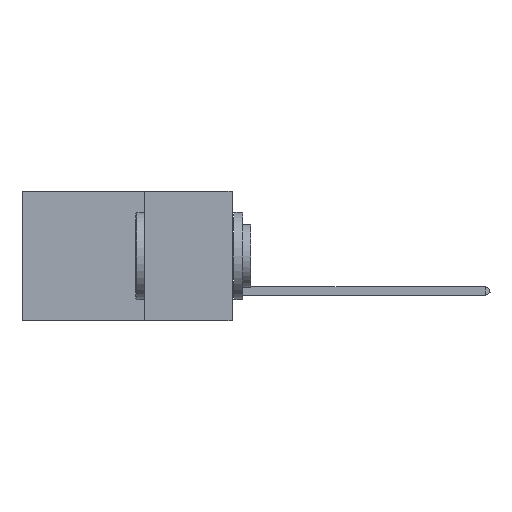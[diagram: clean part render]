
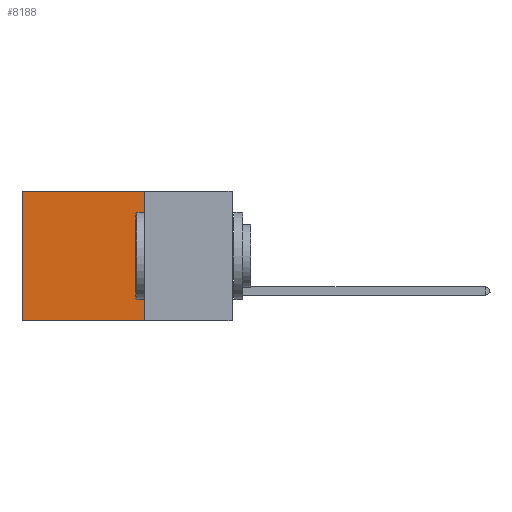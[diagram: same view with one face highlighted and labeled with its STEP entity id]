
A CAD part, left-side view. The second image highlights one B-rep face of the part: STEP entity #8188.
In plain terms, the highlighted planar face has unit normal (-1, 0, 0).
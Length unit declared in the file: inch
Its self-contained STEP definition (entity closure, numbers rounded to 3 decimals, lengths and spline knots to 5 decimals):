
#636 = DIRECTION ( 'NONE',  ( 1., 0., 0. ) ) ;
#708 = DIRECTION ( 'NONE',  ( 0., 1., 0. ) ) ;
#916 = VECTOR ( 'NONE', #20305, 39.37008 ) ;
#1204 = FACE_OUTER_BOUND ( 'NONE', #7259, .T. ) ;
#2306 = LINE ( 'NONE', #9279, #916 ) ;
#2474 = VERTEX_POINT ( 'NONE', #20411 ) ;
#2557 = ORIENTED_EDGE ( 'NONE', *, *, #8892, .F. ) ;
#2837 = CARTESIAN_POINT ( 'NONE',  ( 0.2875, 0.6, -0.37 ) ) ;
#4544 = ORIENTED_EDGE ( 'NONE', *, *, #14849, .T. ) ;
#5032 = DIRECTION ( 'NONE',  ( 0., 1., 0. ) ) ;
#5223 = EDGE_CURVE ( 'NONE', #19744, #2474, #18681, .T. ) ;
#5583 = CARTESIAN_POINT ( 'NONE',  ( 0.2875, 0.25, 0. ) ) ;
#6384 = AXIS2_PLACEMENT_3D ( 'NONE', #8786, #636, #11746 ) ;
#6830 = VERTEX_POINT ( 'NONE', #2837 ) ;
#7013 = PLANE ( 'NONE',  #6384 ) ;
#7259 = EDGE_LOOP ( 'NONE', ( #4544, #13250, #2557, #17634 ) ) ;
#8156 = EDGE_CURVE ( 'NONE', #17563, #6830, #22712, .T. ) ;
#8188 = ADVANCED_FACE ( 'NONE', ( #1204 ), #7013, .F. ) ;
#8786 = CARTESIAN_POINT ( 'NONE',  ( 0.2875, 0.25, 0. ) ) ;
#8892 = EDGE_CURVE ( 'NONE', #19744, #17563, #19636, .T. ) ;
#8899 = DIRECTION ( 'NONE',  ( 0., 0., -1. ) ) ;
#9279 = CARTESIAN_POINT ( 'NONE',  ( 0.2875, 0.6, 0. ) ) ;
#10733 = VECTOR ( 'NONE', #708, 39.37008 ) ;
#10824 = CARTESIAN_POINT ( 'NONE',  ( 0.2875, 0.25, 0. ) ) ;
#11746 = DIRECTION ( 'NONE',  ( 0., 0., -1. ) ) ;
#13250 = ORIENTED_EDGE ( 'NONE', *, *, #8156, .F. ) ;
#14849 = EDGE_CURVE ( 'NONE', #2474, #6830, #2306, .T. ) ;
#16206 = CARTESIAN_POINT ( 'NONE',  ( 0.2875, 0.25, 0. ) ) ;
#16898 = VECTOR ( 'NONE', #8899, 39.37008 ) ;
#17563 = VERTEX_POINT ( 'NONE', #21113 ) ;
#17634 = ORIENTED_EDGE ( 'NONE', *, *, #5223, .T. ) ;
#18681 = LINE ( 'NONE', #16206, #10733 ) ;
#19636 = LINE ( 'NONE', #5583, #16898 ) ;
#19744 = VERTEX_POINT ( 'NONE', #10824 ) ;
#20305 = DIRECTION ( 'NONE',  ( 0., 0., -1. ) ) ;
#20411 = CARTESIAN_POINT ( 'NONE',  ( 0.2875, 0.6, 0. ) ) ;
#20859 = CARTESIAN_POINT ( 'NONE',  ( 0.2875, 0.25, -0.37 ) ) ;
#21113 = CARTESIAN_POINT ( 'NONE',  ( 0.2875, 0.25, -0.37 ) ) ;
#22417 = VECTOR ( 'NONE', #5032, 39.37008 ) ;
#22712 = LINE ( 'NONE', #20859, #22417 ) ;
